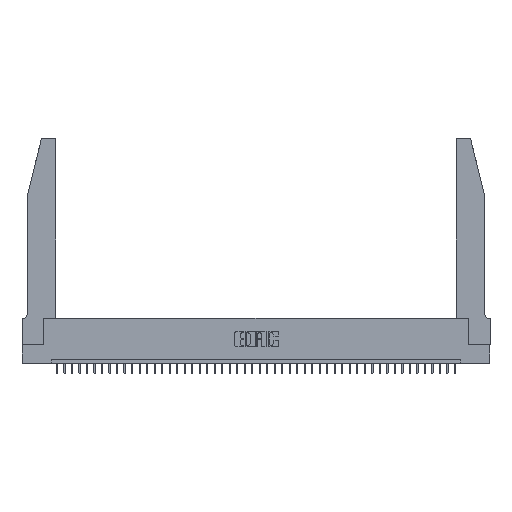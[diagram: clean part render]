
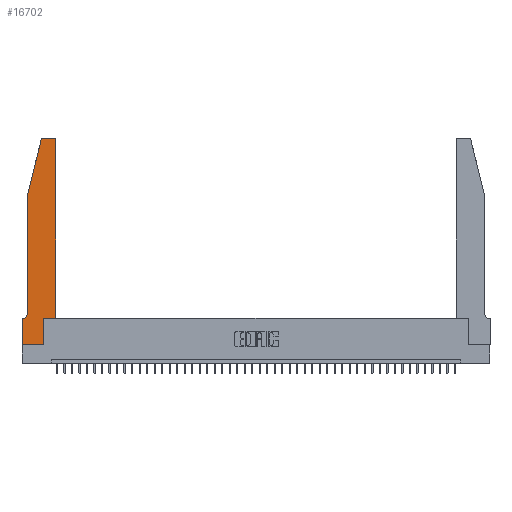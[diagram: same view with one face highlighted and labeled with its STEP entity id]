
A CAD part, top view. The second image highlights one B-rep face of the part: STEP entity #16702.
In plain terms, the highlighted planar face has unit normal (0, 0, 1).
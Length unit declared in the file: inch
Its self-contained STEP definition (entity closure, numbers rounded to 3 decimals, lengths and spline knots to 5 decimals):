
#254 = ORIENTED_EDGE ( 'NONE', *, *, #35072, .T. ) ;
#361 = CARTESIAN_POINT ( 'NONE',  ( 0.0755, 0.35, 0.37 ) ) ;
#365 = CARTESIAN_POINT ( 'NONE',  ( 0.0055, 0.35, 0.37 ) ) ;
#1013 = LINE ( 'NONE', #1460, #18721 ) ;
#1066 = LINE ( 'NONE', #28130, #40872 ) ;
#1460 = CARTESIAN_POINT ( 'NONE',  ( 0.4505, 0.35, 0.37 ) ) ;
#2017 = DIRECTION ( 'NONE',  ( 0., 0., 1. ) ) ;
#2570 = VERTEX_POINT ( 'NONE', #39981 ) ;
#3200 = EDGE_CURVE ( 'NONE', #17968, #16432, #7060, .T. ) ;
#3415 = ORIENTED_EDGE ( 'NONE', *, *, #3200, .T. ) ;
#4287 = VERTEX_POINT ( 'NONE', #5588 ) ;
#4583 = DIRECTION ( 'NONE',  ( 0., -1., 0. ) ) ;
#5588 = CARTESIAN_POINT ( 'NONE',  ( 0.4505, 0.35, 0.37 ) ) ;
#5884 = VECTOR ( 'NONE', #21457, 39.37008 ) ;
#6310 = VECTOR ( 'NONE', #20542, 39.37008 ) ;
#6551 = EDGE_CURVE ( 'NONE', #26740, #42099, #28756, .T. ) ;
#7044 = LINE ( 'NONE', #361, #6310 ) ;
#7060 = LINE ( 'NONE', #11483, #25845 ) ;
#7157 = CARTESIAN_POINT ( 'NONE',  ( 0.2865, 0., 0.37 ) ) ;
#7520 = AXIS2_PLACEMENT_3D ( 'NONE', #26166, #2017, #25530 ) ;
#7972 = ORIENTED_EDGE ( 'NONE', *, *, #27373, .T. ) ;
#8087 = DIRECTION ( 'NONE',  ( 0., 1., 0. ) ) ;
#8656 = CARTESIAN_POINT ( 'NONE',  ( 0.4205, 2.72, 0.37 ) ) ;
#8718 = AXIS2_PLACEMENT_3D ( 'NONE', #8656, #34640, #31936 ) ;
#11123 = CIRCLE ( 'NONE', #23146, 0.03 ) ;
#11378 = CARTESIAN_POINT ( 'NONE',  ( 0.4505, 2.72, 0.37 ) ) ;
#11426 = CARTESIAN_POINT ( 'NONE',  ( 0.2865, 0.35, 0.37 ) ) ;
#11483 = CARTESIAN_POINT ( 'NONE',  ( 0., 0., 0.37 ) ) ;
#12117 = CARTESIAN_POINT ( 'NONE',  ( 0.0755, 0.42, 0.37 ) ) ;
#12161 = DIRECTION ( 'NONE',  ( 0., 0., 1. ) ) ;
#13859 = CARTESIAN_POINT ( 'NONE',  ( 0., 0.35, 0.37 ) ) ;
#15428 = EDGE_CURVE ( 'NONE', #18169, #17298, #32882, .T. ) ;
#15835 = ORIENTED_EDGE ( 'NONE', *, *, #39357, .T. ) ;
#16432 = VERTEX_POINT ( 'NONE', #7157 ) ;
#16702 = ADVANCED_FACE ( 'NONE', ( #39481 ), #39064, .T. ) ;
#16790 = DIRECTION ( 'NONE',  ( 0., -1., 0. ) ) ;
#17298 = VERTEX_POINT ( 'NONE', #365 ) ;
#17675 = VECTOR ( 'NONE', #8087, 39.37008 ) ;
#17968 = VERTEX_POINT ( 'NONE', #40754 ) ;
#18169 = VERTEX_POINT ( 'NONE', #12117 ) ;
#18721 = VECTOR ( 'NONE', #31619, 39.37008 ) ;
#18828 = CARTESIAN_POINT ( 'NONE',  ( 0.0755, 2., 0.37 ) ) ;
#19257 = CARTESIAN_POINT ( 'NONE',  ( 0.4205, 2.75, 0.37 ) ) ;
#20542 = DIRECTION ( 'NONE',  ( -1., 0., 0. ) ) ;
#21008 = ORIENTED_EDGE ( 'NONE', *, *, #15428, .T. ) ;
#21107 = DIRECTION ( 'NONE',  ( -1., 0., 0. ) ) ;
#21399 = VERTEX_POINT ( 'NONE', #11378 ) ;
#21420 = LINE ( 'NONE', #24304, #42151 ) ;
#21457 = DIRECTION ( 'NONE',  ( -1., 0., 0. ) ) ;
#22360 = EDGE_CURVE ( 'NONE', #17298, #30508, #7044, .T. ) ;
#22482 = LINE ( 'NONE', #32700, #5884 ) ;
#23146 = AXIS2_PLACEMENT_3D ( 'NONE', #35675, #12161, #28563 ) ;
#23972 = ORIENTED_EDGE ( 'NONE', *, *, #32689, .T. ) ;
#24137 = ORIENTED_EDGE ( 'NONE', *, *, #33099, .T. ) ;
#24304 = CARTESIAN_POINT ( 'NONE',  ( 0.0755, 2., 0.37 ) ) ;
#24506 = ORIENTED_EDGE ( 'NONE', *, *, #39405, .T. ) ;
#24775 = ORIENTED_EDGE ( 'NONE', *, *, #22360, .T. ) ;
#25454 = CARTESIAN_POINT ( 'NONE',  ( 0.0755, 2., 0.37 ) ) ;
#25530 = DIRECTION ( 'NONE',  ( 1., 0., 0. ) ) ;
#25845 = VECTOR ( 'NONE', #41884, 39.37008 ) ;
#26084 = DIRECTION ( 'NONE',  ( -0.239, -0.971, 0. ) ) ;
#26166 = CARTESIAN_POINT ( 'NONE',  ( 0., 0.35, 0.37 ) ) ;
#26602 = ORIENTED_EDGE ( 'NONE', *, *, #29404, .T. ) ;
#26740 = VERTEX_POINT ( 'NONE', #40548 ) ;
#27373 = EDGE_CURVE ( 'NONE', #16432, #41667, #35584, .T. ) ;
#27824 = CIRCLE ( 'NONE', #8718, 0.03 ) ;
#28130 = CARTESIAN_POINT ( 'NONE',  ( 0.4505, 0.35, 0.37 ) ) ;
#28563 = DIRECTION ( 'NONE',  ( 1., 0., 0. ) ) ;
#28645 = AXIS2_PLACEMENT_3D ( 'NONE', #31956, #41303, #21107 ) ;
#28756 = LINE ( 'NONE', #25454, #35299 ) ;
#29404 = EDGE_CURVE ( 'NONE', #30508, #17968, #36119, .T. ) ;
#30508 = VERTEX_POINT ( 'NONE', #13859 ) ;
#31270 = EDGE_LOOP ( 'NONE', ( #24137, #24506, #42567, #38965, #21008, #24775, #26602, #3415, #7972, #254, #15835, #23972 ) ) ;
#31619 = DIRECTION ( 'NONE',  ( 1., 0., 0. ) ) ;
#31936 = DIRECTION ( 'NONE',  ( 1., 0., 0. ) ) ;
#31956 = CARTESIAN_POINT ( 'NONE',  ( 0.0055, 0.42, 0.37 ) ) ;
#32689 = EDGE_CURVE ( 'NONE', #21399, #37748, #27824, .T. ) ;
#32700 = CARTESIAN_POINT ( 'NONE',  ( 0.2605, 2.75, 0.37 ) ) ;
#32882 = CIRCLE ( 'NONE', #28645, 0.07 ) ;
#33099 = EDGE_CURVE ( 'NONE', #37748, #2570, #22482, .T. ) ;
#33301 = CARTESIAN_POINT ( 'NONE',  ( 0.2865, 0.35, 0.37 ) ) ;
#34640 = DIRECTION ( 'NONE',  ( 0., 0., 1. ) ) ;
#35072 = EDGE_CURVE ( 'NONE', #41667, #4287, #1013, .T. ) ;
#35158 = EDGE_CURVE ( 'NONE', #42099, #18169, #21420, .T. ) ;
#35299 = VECTOR ( 'NONE', #26084, 39.37008 ) ;
#35584 = LINE ( 'NONE', #11426, #17675 ) ;
#35675 = CARTESIAN_POINT ( 'NONE',  ( 0.284, 2.72, 0.37 ) ) ;
#36119 = LINE ( 'NONE', #39867, #41922 ) ;
#37748 = VERTEX_POINT ( 'NONE', #19257 ) ;
#38965 = ORIENTED_EDGE ( 'NONE', *, *, #35158, .T. ) ;
#39064 = PLANE ( 'NONE',  #7520 ) ;
#39357 = EDGE_CURVE ( 'NONE', #4287, #21399, #1066, .T. ) ;
#39405 = EDGE_CURVE ( 'NONE', #2570, #26740, #11123, .T. ) ;
#39481 = FACE_OUTER_BOUND ( 'NONE', #31270, .T. ) ;
#39867 = CARTESIAN_POINT ( 'NONE',  ( 0., 0., 0.37 ) ) ;
#39981 = CARTESIAN_POINT ( 'NONE',  ( 0.284, 2.75, 0.37 ) ) ;
#40548 = CARTESIAN_POINT ( 'NONE',  ( 0.25487, 2.72718, 0.37 ) ) ;
#40754 = CARTESIAN_POINT ( 'NONE',  ( 0., 0., 0.37 ) ) ;
#40872 = VECTOR ( 'NONE', #41698, 39.37008 ) ;
#41303 = DIRECTION ( 'NONE',  ( 0., 0., -1. ) ) ;
#41667 = VERTEX_POINT ( 'NONE', #33301 ) ;
#41698 = DIRECTION ( 'NONE',  ( 0., 1., 0. ) ) ;
#41884 = DIRECTION ( 'NONE',  ( 1., 0., 0. ) ) ;
#41922 = VECTOR ( 'NONE', #16790, 39.37008 ) ;
#42099 = VERTEX_POINT ( 'NONE', #18828 ) ;
#42151 = VECTOR ( 'NONE', #4583, 39.37008 ) ;
#42567 = ORIENTED_EDGE ( 'NONE', *, *, #6551, .T. ) ;
